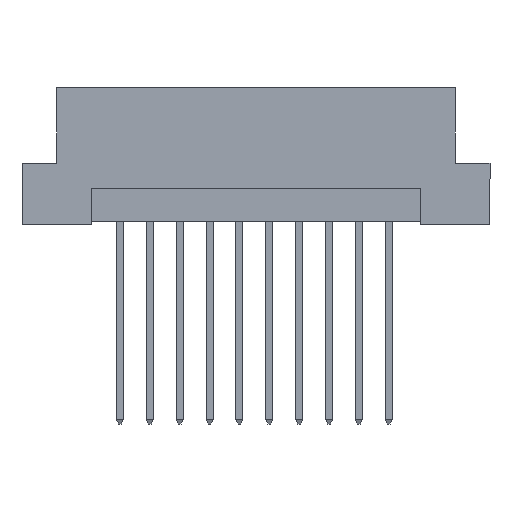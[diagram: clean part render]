
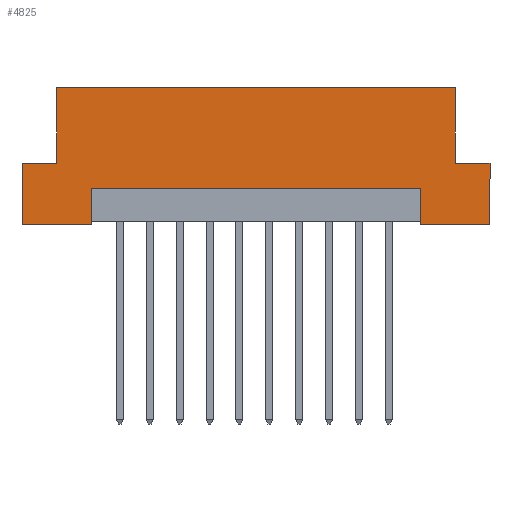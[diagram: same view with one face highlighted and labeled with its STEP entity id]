
A CAD part, front view. The second image highlights one B-rep face of the part: STEP entity #4825.
In plain terms, the highlighted planar face has unit normal (0, -1, 0).
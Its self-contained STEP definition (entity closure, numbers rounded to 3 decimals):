
#41 = CARTESIAN_POINT ( 'NONE',  ( 16.94, -4.3, 11.6 ) ) ;
#99 = CARTESIAN_POINT ( 'NONE',  ( -19.9, -4.3, 5.2 ) ) ;
#177 = VERTEX_POINT ( 'NONE', #989 ) ;
#193 = ORIENTED_EDGE ( 'NONE', *, *, #384, .T. ) ;
#228 = EDGE_CURVE ( 'NONE', #992, #4910, #821, .T. ) ;
#277 = CARTESIAN_POINT ( 'NONE',  ( -16.94, -4.3, 5.2 ) ) ;
#384 = EDGE_CURVE ( 'NONE', #4740, #2003, #3678, .T. ) ;
#419 = CARTESIAN_POINT ( 'NONE',  ( 19.9, -4.3, 0. ) ) ;
#454 = CARTESIAN_POINT ( 'NONE',  ( 19.9, -4.3, 11.6 ) ) ;
#485 = FACE_OUTER_BOUND ( 'NONE', #2467, .T. ) ;
#495 = ORIENTED_EDGE ( 'NONE', *, *, #3833, .F. ) ;
#595 = DIRECTION ( 'NONE',  ( 1., 0., 0. ) ) ;
#597 = VECTOR ( 'NONE', #3690, 1000. ) ;
#601 = ORIENTED_EDGE ( 'NONE', *, *, #3598, .F. ) ;
#645 = CARTESIAN_POINT ( 'NONE',  ( 19.9, -4.3, 11.6 ) ) ;
#681 = DIRECTION ( 'NONE',  ( 1., 0., 0. ) ) ;
#806 = ORIENTED_EDGE ( 'NONE', *, *, #3254, .F. ) ;
#813 = VECTOR ( 'NONE', #4011, 1000. ) ;
#821 = LINE ( 'NONE', #4355, #3706 ) ;
#835 = ORIENTED_EDGE ( 'NONE', *, *, #228, .F. ) ;
#967 = VECTOR ( 'NONE', #1123, 1000. ) ;
#989 = CARTESIAN_POINT ( 'NONE',  ( 19.9, -4.3, 5.2 ) ) ;
#992 = VERTEX_POINT ( 'NONE', #4040 ) ;
#1110 = VERTEX_POINT ( 'NONE', #3418 ) ;
#1123 = DIRECTION ( 'NONE',  ( 1., 0., 0. ) ) ;
#1308 = AXIS2_PLACEMENT_3D ( 'NONE', #3629, #4856, #1673 ) ;
#1321 = ORIENTED_EDGE ( 'NONE', *, *, #3396, .T. ) ;
#1454 = ORIENTED_EDGE ( 'NONE', *, *, #3961, .F. ) ;
#1594 = LINE ( 'NONE', #5092, #3945 ) ;
#1631 = ORIENTED_EDGE ( 'NONE', *, *, #2832, .T. ) ;
#1664 = VECTOR ( 'NONE', #3427, 1000. ) ;
#1673 = DIRECTION ( 'NONE',  ( -1., 0., 0. ) ) ;
#1716 = EDGE_CURVE ( 'NONE', #2003, #4910, #3404, .T. ) ;
#1761 = LINE ( 'NONE', #3987, #597 ) ;
#1846 = CARTESIAN_POINT ( 'NONE',  ( -19.9, -4.3, 5.2 ) ) ;
#1853 = CARTESIAN_POINT ( 'NONE',  ( 19.9, -4.3, 0. ) ) ;
#2003 = VERTEX_POINT ( 'NONE', #4138 ) ;
#2058 = PLANE ( 'NONE',  #1308 ) ;
#2096 = EDGE_CURVE ( 'NONE', #992, #1110, #1761, .T. ) ;
#2139 = CARTESIAN_POINT ( 'NONE',  ( 19.9, -4.3, 5.2 ) ) ;
#2184 = CARTESIAN_POINT ( 'NONE',  ( -14., -4.3, 0. ) ) ;
#2335 = CARTESIAN_POINT ( 'NONE',  ( -16.94, -4.3, 11.6 ) ) ;
#2361 = VERTEX_POINT ( 'NONE', #2335 ) ;
#2406 = DIRECTION ( 'NONE',  ( 0., 0., -1. ) ) ;
#2467 = EDGE_LOOP ( 'NONE', ( #3130, #806, #1631, #495, #3830, #1321, #3738, #1454, #601, #193, #4546, #835 ) ) ;
#2700 = EDGE_CURVE ( 'NONE', #2361, #3222, #4948, .T. ) ;
#2832 = EDGE_CURVE ( 'NONE', #3353, #3273, #4357, .T. ) ;
#2860 = VECTOR ( 'NONE', #681, 1000. ) ;
#2916 = CARTESIAN_POINT ( 'NONE',  ( -19.9, -4.3, 11.6 ) ) ;
#2959 = VECTOR ( 'NONE', #595, 1000. ) ;
#3130 = ORIENTED_EDGE ( 'NONE', *, *, #2096, .T. ) ;
#3146 = CARTESIAN_POINT ( 'NONE',  ( 19.9, -4.3, 0. ) ) ;
#3222 = VERTEX_POINT ( 'NONE', #41 ) ;
#3254 = EDGE_CURVE ( 'NONE', #3353, #1110, #1594, .T. ) ;
#3264 = CARTESIAN_POINT ( 'NONE',  ( 16.94, -4.3, 5.2 ) ) ;
#3273 = VERTEX_POINT ( 'NONE', #3146 ) ;
#3353 = VERTEX_POINT ( 'NONE', #4775 ) ;
#3393 = DIRECTION ( 'NONE',  ( 0., 0., 1. ) ) ;
#3396 = EDGE_CURVE ( 'NONE', #5020, #3222, #4421, .T. ) ;
#3404 = LINE ( 'NONE', #1853, #1664 ) ;
#3418 = CARTESIAN_POINT ( 'NONE',  ( 14., -4.3, 3. ) ) ;
#3427 = DIRECTION ( 'NONE',  ( 1., 0., 0. ) ) ;
#3448 = VECTOR ( 'NONE', #3393, 1000. ) ;
#3560 = VERTEX_POINT ( 'NONE', #277 ) ;
#3575 = LINE ( 'NONE', #454, #4780 ) ;
#3598 = EDGE_CURVE ( 'NONE', #4740, #3560, #3780, .T. ) ;
#3626 = VECTOR ( 'NONE', #4136, 1000. ) ;
#3629 = CARTESIAN_POINT ( 'NONE',  ( 19.9, -4.3, 11.6 ) ) ;
#3678 = LINE ( 'NONE', #2916, #3626 ) ;
#3690 = DIRECTION ( 'NONE',  ( 1., 0., 0. ) ) ;
#3692 = CARTESIAN_POINT ( 'NONE',  ( -16.94, -4.3, 5.2 ) ) ;
#3706 = VECTOR ( 'NONE', #2406, 1000. ) ;
#3738 = ORIENTED_EDGE ( 'NONE', *, *, #2700, .F. ) ;
#3780 = LINE ( 'NONE', #1846, #2860 ) ;
#3830 = ORIENTED_EDGE ( 'NONE', *, *, #4256, .F. ) ;
#3833 = EDGE_CURVE ( 'NONE', #177, #3273, #3575, .T. ) ;
#3852 = VECTOR ( 'NONE', #4155, 1000. ) ;
#3945 = VECTOR ( 'NONE', #4347, 1000. ) ;
#3961 = EDGE_CURVE ( 'NONE', #3560, #2361, #4960, .T. ) ;
#3987 = CARTESIAN_POINT ( 'NONE',  ( -14., -4.3, 3. ) ) ;
#4011 = DIRECTION ( 'NONE',  ( 0., 0., 1. ) ) ;
#4040 = CARTESIAN_POINT ( 'NONE',  ( -14., -4.3, 3. ) ) ;
#4136 = DIRECTION ( 'NONE',  ( 0., 0., -1. ) ) ;
#4138 = CARTESIAN_POINT ( 'NONE',  ( -19.9, -4.3, 0. ) ) ;
#4155 = DIRECTION ( 'NONE',  ( 1., 0., 0. ) ) ;
#4256 = EDGE_CURVE ( 'NONE', #5020, #177, #4888, .T. ) ;
#4347 = DIRECTION ( 'NONE',  ( 0., 0., 1. ) ) ;
#4355 = CARTESIAN_POINT ( 'NONE',  ( -14., -4.3, 0.2 ) ) ;
#4357 = LINE ( 'NONE', #419, #967 ) ;
#4416 = DIRECTION ( 'NONE',  ( 0., 0., -1. ) ) ;
#4421 = LINE ( 'NONE', #3264, #813 ) ;
#4546 = ORIENTED_EDGE ( 'NONE', *, *, #1716, .T. ) ;
#4740 = VERTEX_POINT ( 'NONE', #99 ) ;
#4775 = CARTESIAN_POINT ( 'NONE',  ( 14., -4.3, 0. ) ) ;
#4780 = VECTOR ( 'NONE', #4416, 1000. ) ;
#4825 = ADVANCED_FACE ( 'NONE', ( #485 ), #2058, .F. ) ;
#4856 = DIRECTION ( 'NONE',  ( 0., 1., 0. ) ) ;
#4888 = LINE ( 'NONE', #2139, #2959 ) ;
#4910 = VERTEX_POINT ( 'NONE', #2184 ) ;
#4948 = LINE ( 'NONE', #645, #3852 ) ;
#4960 = LINE ( 'NONE', #3692, #3448 ) ;
#5020 = VERTEX_POINT ( 'NONE', #5067 ) ;
#5067 = CARTESIAN_POINT ( 'NONE',  ( 16.94, -4.3, 5.2 ) ) ;
#5092 = CARTESIAN_POINT ( 'NONE',  ( 14., -4.3, 0.2 ) ) ;
